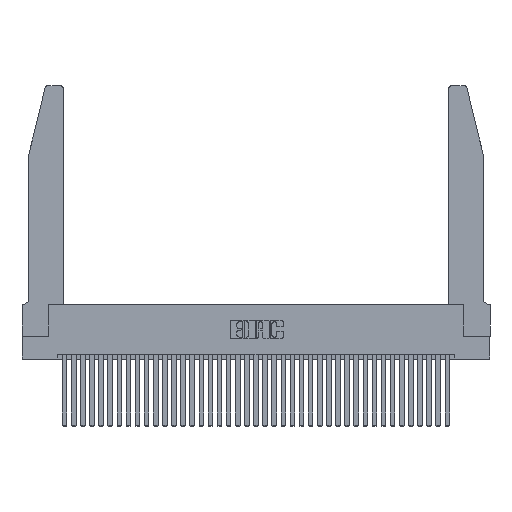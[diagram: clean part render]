
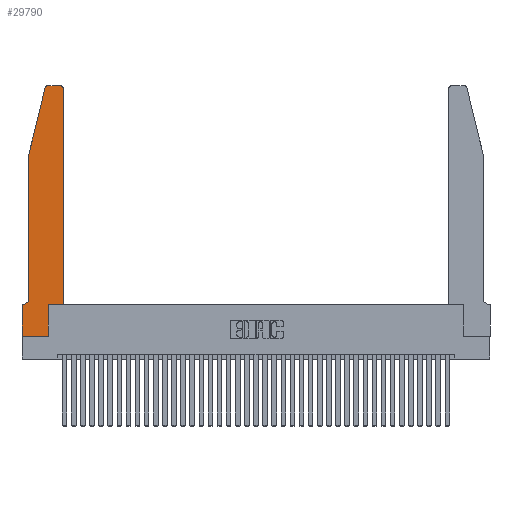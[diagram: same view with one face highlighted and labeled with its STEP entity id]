
A CAD part, top view. The second image highlights one B-rep face of the part: STEP entity #29790.
In plain terms, the highlighted planar face has unit normal (0, 0, 1).
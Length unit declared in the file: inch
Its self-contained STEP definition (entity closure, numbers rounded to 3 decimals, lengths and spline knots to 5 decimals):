
#933 = VECTOR ( 'NONE', #17186, 39.37008 ) ;
#1196 = EDGE_CURVE ( 'NONE', #15156, #29870, #24500, .T. ) ;
#1736 = CARTESIAN_POINT ( 'NONE',  ( 0.284, 2.75, 0.37 ) ) ;
#1810 = DIRECTION ( 'NONE',  ( 1., 0., 0. ) ) ;
#2081 = LINE ( 'NONE', #7023, #22823 ) ;
#3478 = CARTESIAN_POINT ( 'NONE',  ( 0.2865, 0.35, 0.37 ) ) ;
#4094 = ORIENTED_EDGE ( 'NONE', *, *, #9642, .T. ) ;
#4692 = ORIENTED_EDGE ( 'NONE', *, *, #5433, .T. ) ;
#5433 = EDGE_CURVE ( 'NONE', #29870, #13699, #24472, .T. ) ;
#5451 = CARTESIAN_POINT ( 'NONE',  ( 0., 0., 0.37 ) ) ;
#5732 = CARTESIAN_POINT ( 'NONE',  ( 0.2865, 0., 0.37 ) ) ;
#5930 = VERTEX_POINT ( 'NONE', #23824 ) ;
#6248 = VECTOR ( 'NONE', #21081, 39.37008 ) ;
#6331 = EDGE_CURVE ( 'NONE', #23221, #5930, #21666, .T. ) ;
#6622 = CIRCLE ( 'NONE', #31874, 0.07 ) ;
#7023 = CARTESIAN_POINT ( 'NONE',  ( 0.4505, 0.35, 0.37 ) ) ;
#8766 = DIRECTION ( 'NONE',  ( 1., 0., 0. ) ) ;
#9323 = ORIENTED_EDGE ( 'NONE', *, *, #28125, .T. ) ;
#9642 = EDGE_CURVE ( 'NONE', #5930, #35677, #20094, .T. ) ;
#9756 = VECTOR ( 'NONE', #26933, 39.37008 ) ;
#10306 = ORIENTED_EDGE ( 'NONE', *, *, #38133, .T. ) ;
#10781 = CARTESIAN_POINT ( 'NONE',  ( 0.0755, 0.42, 0.37 ) ) ;
#10869 = CARTESIAN_POINT ( 'NONE',  ( 0.4505, 0.35, 0.37 ) ) ;
#11292 = DIRECTION ( 'NONE',  ( 1., 0., 0. ) ) ;
#11407 = CARTESIAN_POINT ( 'NONE',  ( 0., 0., 0.37 ) ) ;
#11485 = CARTESIAN_POINT ( 'NONE',  ( 0., 0., 0.37 ) ) ;
#11565 = DIRECTION ( 'NONE',  ( 1., 0., 0. ) ) ;
#11701 = LINE ( 'NONE', #15843, #32458 ) ;
#12012 = VECTOR ( 'NONE', #35466, 39.37008 ) ;
#12209 = CARTESIAN_POINT ( 'NONE',  ( 0.0055, 0.42, 0.37 ) ) ;
#12228 = ORIENTED_EDGE ( 'NONE', *, *, #34906, .T. ) ;
#12589 = VECTOR ( 'NONE', #21576, 39.37008 ) ;
#13593 = ORIENTED_EDGE ( 'NONE', *, *, #18709, .T. ) ;
#13699 = VERTEX_POINT ( 'NONE', #34545 ) ;
#13761 = CARTESIAN_POINT ( 'NONE',  ( 0., 0.35, 0.37 ) ) ;
#13861 = CIRCLE ( 'NONE', #23708, 0.03 ) ;
#15156 = VERTEX_POINT ( 'NONE', #5732 ) ;
#15288 = VERTEX_POINT ( 'NONE', #10781 ) ;
#15843 = CARTESIAN_POINT ( 'NONE',  ( 0.0755, 2., 0.37 ) ) ;
#16354 = VERTEX_POINT ( 'NONE', #13761 ) ;
#16472 = EDGE_CURVE ( 'NONE', #25257, #15156, #21470, .T. ) ;
#16559 = ORIENTED_EDGE ( 'NONE', *, *, #16472, .T. ) ;
#17186 = DIRECTION ( 'NONE',  ( 1., 0., 0. ) ) ;
#17689 = DIRECTION ( 'NONE',  ( 0., 0., 1. ) ) ;
#17948 = CARTESIAN_POINT ( 'NONE',  ( 0.4205, 2.72, 0.37 ) ) ;
#18014 = ORIENTED_EDGE ( 'NONE', *, *, #32966, .T. ) ;
#18709 = EDGE_CURVE ( 'NONE', #23089, #30043, #36081, .T. ) ;
#19919 = PLANE ( 'NONE',  #25680 ) ;
#20094 = LINE ( 'NONE', #32968, #6248 ) ;
#20417 = LINE ( 'NONE', #27382, #12589 ) ;
#21081 = DIRECTION ( 'NONE',  ( -1., 0., 0. ) ) ;
#21297 = VECTOR ( 'NONE', #31626, 39.37008 ) ;
#21470 = LINE ( 'NONE', #11407, #36265 ) ;
#21576 = DIRECTION ( 'NONE',  ( -1., 0., 0. ) ) ;
#21666 = CIRCLE ( 'NONE', #29706, 0.03 ) ;
#22823 = VECTOR ( 'NONE', #30631, 39.37008 ) ;
#22967 = EDGE_LOOP ( 'NONE', ( #4094, #24311, #13593, #12228, #35979, #9323, #10306, #16559, #34888, #4692, #18014, #31900 ) ) ;
#23089 = VERTEX_POINT ( 'NONE', #24692 ) ;
#23184 = CARTESIAN_POINT ( 'NONE',  ( 0.0755, 2., 0.37 ) ) ;
#23221 = VERTEX_POINT ( 'NONE', #31494 ) ;
#23527 = LINE ( 'NONE', #11485, #12012 ) ;
#23708 = AXIS2_PLACEMENT_3D ( 'NONE', #25838, #35029, #11565 ) ;
#23824 = CARTESIAN_POINT ( 'NONE',  ( 0.4205, 2.75, 0.37 ) ) ;
#24311 = ORIENTED_EDGE ( 'NONE', *, *, #29815, .T. ) ;
#24472 = LINE ( 'NONE', #10869, #933 ) ;
#24500 = LINE ( 'NONE', #3478, #9756 ) ;
#24692 = CARTESIAN_POINT ( 'NONE',  ( 0.25487, 2.72718, 0.37 ) ) ;
#24960 = VERTEX_POINT ( 'NONE', #25797 ) ;
#25257 = VERTEX_POINT ( 'NONE', #5451 ) ;
#25662 = CARTESIAN_POINT ( 'NONE',  ( 0.0755, 2., 0.37 ) ) ;
#25680 = AXIS2_PLACEMENT_3D ( 'NONE', #29202, #29083, #11292 ) ;
#25797 = CARTESIAN_POINT ( 'NONE',  ( 0.0055, 0.35, 0.37 ) ) ;
#25838 = CARTESIAN_POINT ( 'NONE',  ( 0.284, 2.72, 0.37 ) ) ;
#25965 = CARTESIAN_POINT ( 'NONE',  ( 0.2865, 0.35, 0.37 ) ) ;
#26933 = DIRECTION ( 'NONE',  ( 0., 1., 0. ) ) ;
#27278 = FACE_OUTER_BOUND ( 'NONE', #22967, .T. ) ;
#27382 = CARTESIAN_POINT ( 'NONE',  ( 0.0755, 0.35, 0.37 ) ) ;
#27707 = DIRECTION ( 'NONE',  ( 0., -1., 0. ) ) ;
#27950 = EDGE_CURVE ( 'NONE', #15288, #24960, #6622, .T. ) ;
#28125 = EDGE_CURVE ( 'NONE', #24960, #16354, #20417, .T. ) ;
#29083 = DIRECTION ( 'NONE',  ( 0., 0., 1. ) ) ;
#29202 = CARTESIAN_POINT ( 'NONE',  ( 0., 0.35, 0.37 ) ) ;
#29706 = AXIS2_PLACEMENT_3D ( 'NONE', #17948, #17689, #8766 ) ;
#29790 = ADVANCED_FACE ( 'NONE', ( #27278 ), #19919, .T. ) ;
#29815 = EDGE_CURVE ( 'NONE', #35677, #23089, #13861, .T. ) ;
#29870 = VERTEX_POINT ( 'NONE', #25965 ) ;
#30043 = VERTEX_POINT ( 'NONE', #23184 ) ;
#30631 = DIRECTION ( 'NONE',  ( 0., 1., 0. ) ) ;
#31494 = CARTESIAN_POINT ( 'NONE',  ( 0.4505, 2.72, 0.37 ) ) ;
#31626 = DIRECTION ( 'NONE',  ( -0.239, -0.971, 0. ) ) ;
#31874 = AXIS2_PLACEMENT_3D ( 'NONE', #12209, #32829, #35664 ) ;
#31900 = ORIENTED_EDGE ( 'NONE', *, *, #6331, .T. ) ;
#32458 = VECTOR ( 'NONE', #27707, 39.37008 ) ;
#32829 = DIRECTION ( 'NONE',  ( 0., 0., -1. ) ) ;
#32966 = EDGE_CURVE ( 'NONE', #13699, #23221, #2081, .T. ) ;
#32968 = CARTESIAN_POINT ( 'NONE',  ( 0.2605, 2.75, 0.37 ) ) ;
#34545 = CARTESIAN_POINT ( 'NONE',  ( 0.4505, 0.35, 0.37 ) ) ;
#34888 = ORIENTED_EDGE ( 'NONE', *, *, #1196, .T. ) ;
#34906 = EDGE_CURVE ( 'NONE', #30043, #15288, #11701, .T. ) ;
#35029 = DIRECTION ( 'NONE',  ( 0., 0., 1. ) ) ;
#35466 = DIRECTION ( 'NONE',  ( 0., -1., 0. ) ) ;
#35664 = DIRECTION ( 'NONE',  ( -1., 0., 0. ) ) ;
#35677 = VERTEX_POINT ( 'NONE', #1736 ) ;
#35979 = ORIENTED_EDGE ( 'NONE', *, *, #27950, .T. ) ;
#36081 = LINE ( 'NONE', #25662, #21297 ) ;
#36265 = VECTOR ( 'NONE', #1810, 39.37008 ) ;
#38133 = EDGE_CURVE ( 'NONE', #16354, #25257, #23527, .T. ) ;
